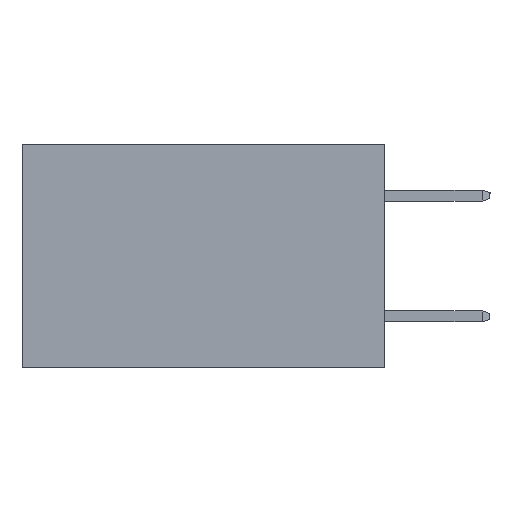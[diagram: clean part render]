
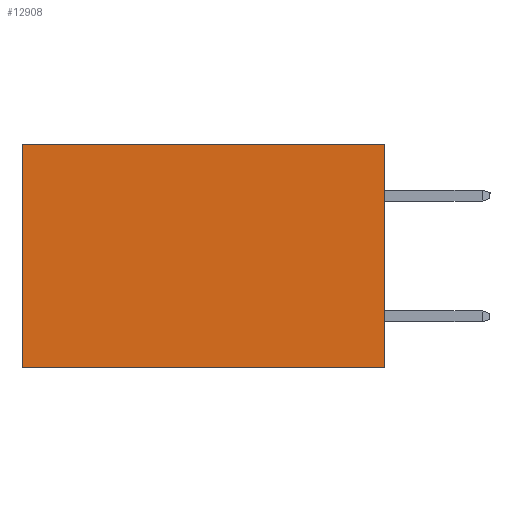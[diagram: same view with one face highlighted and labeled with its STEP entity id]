
A CAD part, left-side view. The second image highlights one B-rep face of the part: STEP entity #12908.
In plain terms, the highlighted planar face has unit normal (-1, 0, 0).
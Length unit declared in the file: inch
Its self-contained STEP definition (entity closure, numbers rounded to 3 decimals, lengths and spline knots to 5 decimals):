
#104 = LINE ( 'NONE', #23075, #22159 ) ;
#904 = ORIENTED_EDGE ( 'NONE', *, *, #9474, .T. ) ;
#1365 = ORIENTED_EDGE ( 'NONE', *, *, #12640, .T. ) ;
#2052 = AXIS2_PLACEMENT_3D ( 'NONE', #19068, #7755, #23190 ) ;
#2884 = CARTESIAN_POINT ( 'NONE',  ( 0.2615, 0., 0. ) ) ;
#3930 = CARTESIAN_POINT ( 'NONE',  ( 0.2615, 0., -0.37 ) ) ;
#3946 = ORIENTED_EDGE ( 'NONE', *, *, #14145, .F. ) ;
#5683 = LINE ( 'NONE', #13604, #22316 ) ;
#5875 = FACE_OUTER_BOUND ( 'NONE', #10706, .T. ) ;
#7755 = DIRECTION ( 'NONE',  ( 1., 0., 0. ) ) ;
#8156 = LINE ( 'NONE', #2884, #14474 ) ;
#8412 = VERTEX_POINT ( 'NONE', #11908 ) ;
#8969 = VECTOR ( 'NONE', #21467, 39.37008 ) ;
#9088 = CARTESIAN_POINT ( 'NONE',  ( 0.2615, 0.6, -0.37 ) ) ;
#9474 = EDGE_CURVE ( 'NONE', #8412, #13147, #5683, .T. ) ;
#10158 = LINE ( 'NONE', #3930, #8969 ) ;
#10706 = EDGE_LOOP ( 'NONE', ( #904, #24121, #3946, #1365 ) ) ;
#11908 = CARTESIAN_POINT ( 'NONE',  ( 0.2615, 0.6, 0. ) ) ;
#12257 = VERTEX_POINT ( 'NONE', #22114 ) ;
#12640 = EDGE_CURVE ( 'NONE', #16606, #8412, #8156, .T. ) ;
#12908 = ADVANCED_FACE ( 'NONE', ( #5875 ), #13545, .F. ) ;
#13147 = VERTEX_POINT ( 'NONE', #9088 ) ;
#13354 = DIRECTION ( 'NONE',  ( 0., 0., -1. ) ) ;
#13419 = CARTESIAN_POINT ( 'NONE',  ( 0.2615, 0., 0. ) ) ;
#13545 = PLANE ( 'NONE',  #2052 ) ;
#13604 = CARTESIAN_POINT ( 'NONE',  ( 0.2615, 0.6, -0.37 ) ) ;
#14145 = EDGE_CURVE ( 'NONE', #16606, #12257, #104, .T. ) ;
#14474 = VECTOR ( 'NONE', #21710, 39.37008 ) ;
#15138 = EDGE_CURVE ( 'NONE', #12257, #13147, #10158, .T. ) ;
#16606 = VERTEX_POINT ( 'NONE', #13419 ) ;
#19068 = CARTESIAN_POINT ( 'NONE',  ( 0.2615, 0., -0.37 ) ) ;
#21467 = DIRECTION ( 'NONE',  ( 0., 1., 0. ) ) ;
#21710 = DIRECTION ( 'NONE',  ( 0., 1., 0. ) ) ;
#22114 = CARTESIAN_POINT ( 'NONE',  ( 0.2615, 0., -0.37 ) ) ;
#22159 = VECTOR ( 'NONE', #23660, 39.37008 ) ;
#22316 = VECTOR ( 'NONE', #13354, 39.37008 ) ;
#23075 = CARTESIAN_POINT ( 'NONE',  ( 0.2615, 0., -0.37 ) ) ;
#23190 = DIRECTION ( 'NONE',  ( 0., 0., -1. ) ) ;
#23660 = DIRECTION ( 'NONE',  ( 0., 0., -1. ) ) ;
#24121 = ORIENTED_EDGE ( 'NONE', *, *, #15138, .F. ) ;
